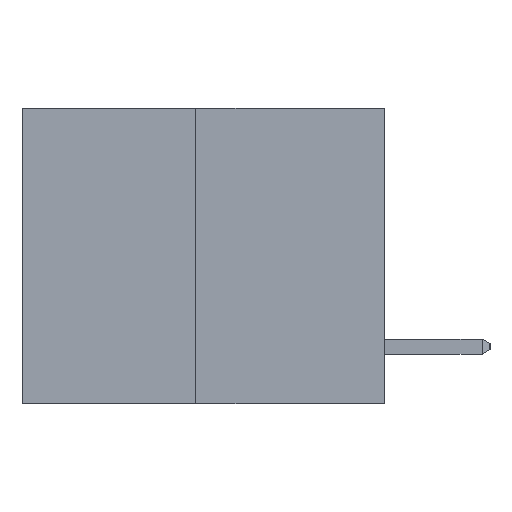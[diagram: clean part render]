
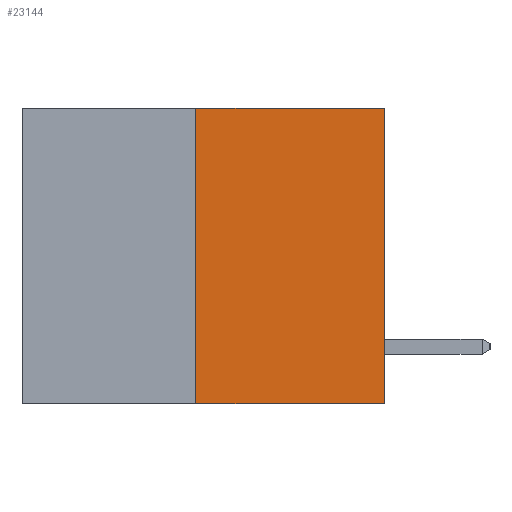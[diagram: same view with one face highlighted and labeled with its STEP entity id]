
A CAD part, left-side view. The second image highlights one B-rep face of the part: STEP entity #23144.
In plain terms, the highlighted planar face has unit normal (-1, 0, 0).
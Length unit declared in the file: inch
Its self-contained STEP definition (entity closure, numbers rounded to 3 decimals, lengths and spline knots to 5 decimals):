
#525 = VECTOR ( 'NONE', #21258, 39.37008 ) ;
#780 = CARTESIAN_POINT ( 'NONE',  ( 0., 0., -0.49 ) ) ;
#859 = VERTEX_POINT ( 'NONE', #16878 ) ;
#1935 = LINE ( 'NONE', #5381, #8041 ) ;
#2814 = CARTESIAN_POINT ( 'NONE',  ( 0., 0.312, -0.49 ) ) ;
#3499 = EDGE_LOOP ( 'NONE', ( #12025, #23646, #17094, #18999 ) ) ;
#5381 = CARTESIAN_POINT ( 'NONE',  ( 0., 0., 0. ) ) ;
#6862 = LINE ( 'NONE', #20299, #8762 ) ;
#6993 = CARTESIAN_POINT ( 'NONE',  ( 0., 0.6, -0.49 ) ) ;
#7342 = CARTESIAN_POINT ( 'NONE',  ( 0., 0.6, 0. ) ) ;
#7428 = EDGE_CURVE ( 'NONE', #859, #15796, #17881, .T. ) ;
#8041 = VECTOR ( 'NONE', #9593, 39.37008 ) ;
#8762 = VECTOR ( 'NONE', #16095, 39.37008 ) ;
#9593 = DIRECTION ( 'NONE',  ( 0., 0., 1. ) ) ;
#11494 = DIRECTION ( 'NONE',  ( 0., 0., -1. ) ) ;
#12025 = ORIENTED_EDGE ( 'NONE', *, *, #18657, .F. ) ;
#13628 = LINE ( 'NONE', #2814, #525 ) ;
#14032 = VERTEX_POINT ( 'NONE', #20688 ) ;
#14846 = EDGE_CURVE ( 'NONE', #15796, #14032, #1935, .T. ) ;
#15008 = AXIS2_PLACEMENT_3D ( 'NONE', #7342, #23507, #11494 ) ;
#15496 = EDGE_CURVE ( 'NONE', #17863, #14032, #6862, .T. ) ;
#15746 = CARTESIAN_POINT ( 'NONE',  ( 0., 0.312, 0. ) ) ;
#15796 = VERTEX_POINT ( 'NONE', #780 ) ;
#16095 = DIRECTION ( 'NONE',  ( 0., -1., 0. ) ) ;
#16878 = CARTESIAN_POINT ( 'NONE',  ( 0., 0.312, -0.49 ) ) ;
#17094 = ORIENTED_EDGE ( 'NONE', *, *, #14846, .T. ) ;
#17340 = DIRECTION ( 'NONE',  ( 0., -1., 0. ) ) ;
#17863 = VERTEX_POINT ( 'NONE', #15746 ) ;
#17881 = LINE ( 'NONE', #6993, #21092 ) ;
#18657 = EDGE_CURVE ( 'NONE', #859, #17863, #13628, .T. ) ;
#18999 = ORIENTED_EDGE ( 'NONE', *, *, #15496, .F. ) ;
#19406 = PLANE ( 'NONE',  #15008 ) ;
#19647 = FACE_OUTER_BOUND ( 'NONE', #3499, .T. ) ;
#20299 = CARTESIAN_POINT ( 'NONE',  ( 0., 0.6, 0. ) ) ;
#20688 = CARTESIAN_POINT ( 'NONE',  ( 0., 0., 0. ) ) ;
#21092 = VECTOR ( 'NONE', #17340, 39.37008 ) ;
#21258 = DIRECTION ( 'NONE',  ( 0., 0., 1. ) ) ;
#23144 = ADVANCED_FACE ( 'NONE', ( #19647 ), #19406, .F. ) ;
#23507 = DIRECTION ( 'NONE',  ( 1., 0., 0. ) ) ;
#23646 = ORIENTED_EDGE ( 'NONE', *, *, #7428, .T. ) ;
